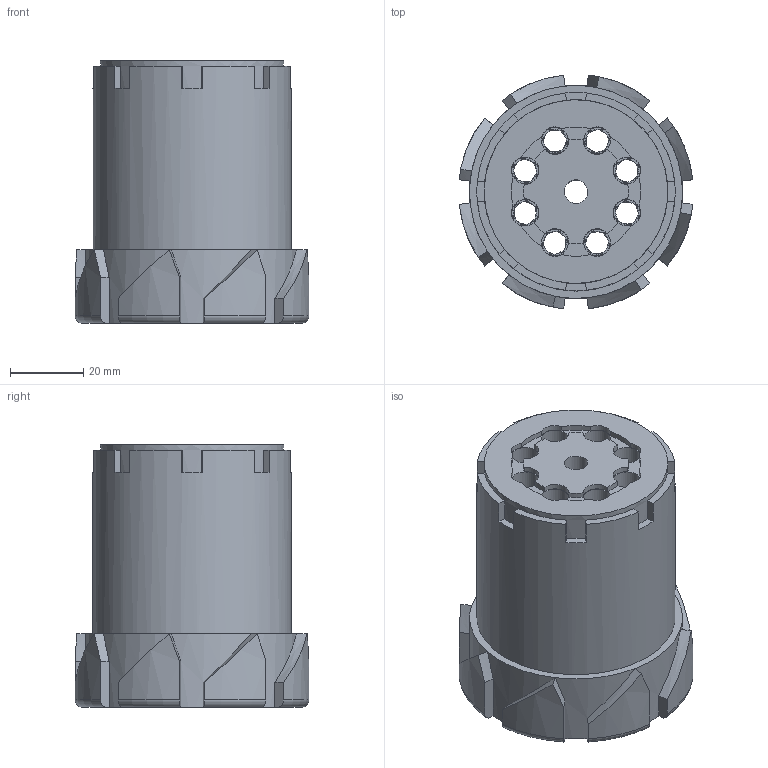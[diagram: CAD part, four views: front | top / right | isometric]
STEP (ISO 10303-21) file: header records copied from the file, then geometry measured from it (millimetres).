
FILE_DESCRIPTION((''),'2;1');
FILE_NAME('PM522INSERTFrontCylinderAssy2.stp','2015-10-01T18:18:11',('JamesRPatrick'),(''),'Autodesk Inventor 2012','Autodesk Inventor 2012','');
FILE_SCHEMA(('AUTOMOTIVE_DESIGN { 1 0 10303 214 1 1 1 1 }'));
Length unit declared in the file: millimetre
Products named in the file (3): PM522INSERTFrontCylinderAssy2.iam (LevelofDetail1); PM522INSERTCylinder2; PM522INSERTFrontIndexRing2
Assembly tree (2 placements, depth 2):
  PM522INSERTFrontCylinderAssy2.iam (LevelofDetail1)
    PM522INSERTCylinder2
    PM522INSERTFrontIndexRing2
Bounding box: 63.65 x 63.65 x 71.5 mm (x, y, z)
Volume: 152188.7 mm3; surface area: 39711.1 mm2
Topology: 2 solids, 2 shells, 258 faces, 717 edges, 473 vertices
Faces by surface type: cylinder 108, bspline 80, plane 62, torus 8
Full cylindrical faces by diameter (mm): 6.4 x1, 7.244 x8, 50 x1, 54 x2
Entity records: 10869 total; most frequent: CARTESIAN_POINT 4563, ORIENTED_EDGE 1404, DIRECTION 1170, EDGE_CURVE 702, AXIS2_PLACEMENT_3D 509, VERTEX_POINT 470, CIRCLE 326, EDGE_LOOP 300
